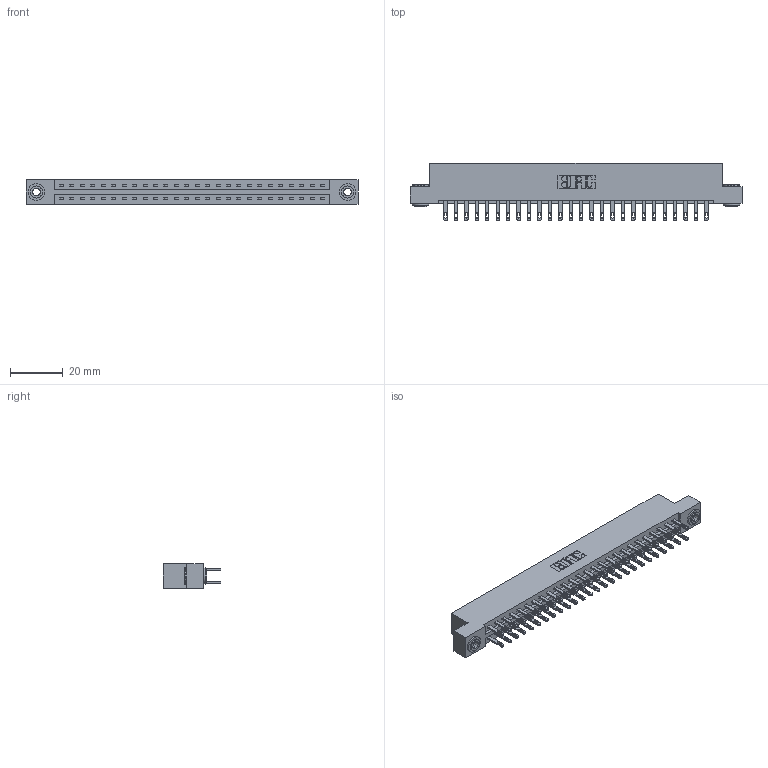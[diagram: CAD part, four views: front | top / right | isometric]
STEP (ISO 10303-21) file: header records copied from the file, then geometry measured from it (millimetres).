
FILE_DESCRIPTION (( 'STEP AP203' ), '1' );
FILE_NAME ('337-052-500-203.STEP', '2019-10-09T16:25:55', ( '' ), ( '' ), 'SwSTEP 2.0', 'SolidWorks 2016', '' );
FILE_SCHEMA (( 'CONFIG_CONTROL_DESIGN' ));
Length unit declared in the file: inch
Products named in the file (4): 337 Part_Flush Mounting Lugs - 0.156 Dia-TH; 345-292-001_345-293-100; 345-250-002_345-250-002-102; 337-052-500-203
Assembly tree (55 placements, depth 2):
  337-052-500-203
    337 Part_Flush Mounting Lugs - 0.156 Dia-TH
    345-292-001_345-293-100  x52
    345-250-002_345-250-002-102  x2
Bounding box: 126.03 x 21.85 x 9.4 mm (x, y, z)
Volume: 13247.9 mm3; surface area: 15622.7 mm2
Topology: 55 solids, 55 shells, 2752 faces, 8343 edges, 5558 vertices
Faces by surface type: plane 1744, cylinder 1000, cone 8
Entity records: 22808 total; most frequent: CARTESIAN_POINT 3829, ORIENTED_EDGE 3758, DIRECTION 3321, EDGE_CURVE 1879, LINE 1723, VECTOR 1723, VERTEX_POINT 1250, AXIS2_PLACEMENT_3D 799
